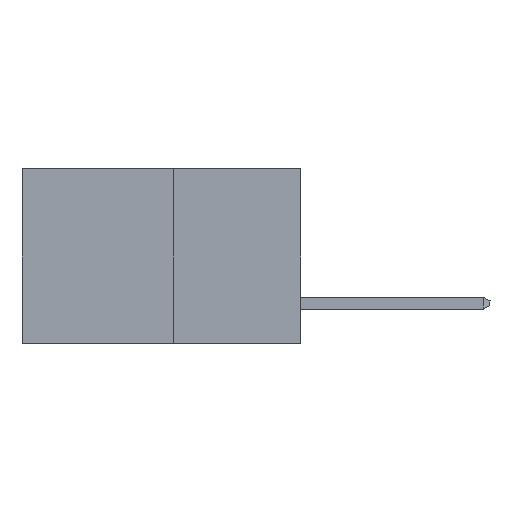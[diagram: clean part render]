
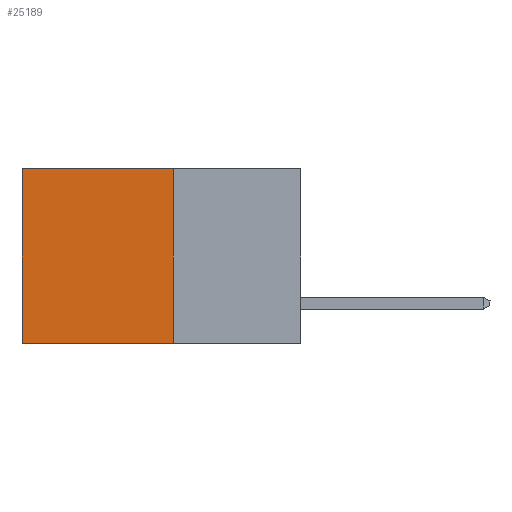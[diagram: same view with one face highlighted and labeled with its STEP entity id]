
A CAD part, left-side view. The second image highlights one B-rep face of the part: STEP entity #25189.
In plain terms, the highlighted planar face has unit normal (-1, 0, 0).
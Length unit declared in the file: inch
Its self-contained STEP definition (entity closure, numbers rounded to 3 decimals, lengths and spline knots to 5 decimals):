
#1989 = CARTESIAN_POINT ( 'NONE',  ( 0.277, 0.27, 0. ) ) ;
#2246 = VERTEX_POINT ( 'NONE', #28020 ) ;
#4218 = LINE ( 'NONE', #16928, #22026 ) ;
#4306 = LINE ( 'NONE', #18485, #16196 ) ;
#4368 = CARTESIAN_POINT ( 'NONE',  ( 0.277, 0.27, -0.37 ) ) ;
#5624 = ORIENTED_EDGE ( 'NONE', *, *, #8021, .F. ) ;
#7954 = DIRECTION ( 'NONE',  ( 0., 1., 0. ) ) ;
#8021 = EDGE_CURVE ( 'NONE', #15554, #9313, #17355, .T. ) ;
#8435 = PLANE ( 'NONE',  #23265 ) ;
#8620 = VERTEX_POINT ( 'NONE', #1989 ) ;
#9313 = VERTEX_POINT ( 'NONE', #13211 ) ;
#9419 = VECTOR ( 'NONE', #7954, 39.37008 ) ;
#10452 = CARTESIAN_POINT ( 'NONE',  ( 0.277, 0.27, -0.37 ) ) ;
#10626 = EDGE_LOOP ( 'NONE', ( #17149, #5624, #13138, #19740 ) ) ;
#10680 = CARTESIAN_POINT ( 'NONE',  ( 0.277, 0.27, -0.37 ) ) ;
#11411 = VECTOR ( 'NONE', #28932, 39.37008 ) ;
#11792 = DIRECTION ( 'NONE',  ( 0., 0., -1. ) ) ;
#12444 = DIRECTION ( 'NONE',  ( 0., 0., -1. ) ) ;
#12917 = DIRECTION ( 'NONE',  ( 1., 0., 0. ) ) ;
#13138 = ORIENTED_EDGE ( 'NONE', *, *, #14913, .F. ) ;
#13211 = CARTESIAN_POINT ( 'NONE',  ( 0.277, 0.59, -0.37 ) ) ;
#14913 = EDGE_CURVE ( 'NONE', #8620, #15554, #4218, .T. ) ;
#15338 = FACE_OUTER_BOUND ( 'NONE', #10626, .T. ) ;
#15554 = VERTEX_POINT ( 'NONE', #10452 ) ;
#16196 = VECTOR ( 'NONE', #11792, 39.37008 ) ;
#16928 = CARTESIAN_POINT ( 'NONE',  ( 0.277, 0.27, -0.37 ) ) ;
#17149 = ORIENTED_EDGE ( 'NONE', *, *, #27931, .T. ) ;
#17355 = LINE ( 'NONE', #4368, #11411 ) ;
#18485 = CARTESIAN_POINT ( 'NONE',  ( 0.277, 0.59, -0.37 ) ) ;
#19740 = ORIENTED_EDGE ( 'NONE', *, *, #21064, .T. ) ;
#20564 = LINE ( 'NONE', #25742, #9419 ) ;
#21064 = EDGE_CURVE ( 'NONE', #8620, #2246, #20564, .T. ) ;
#22026 = VECTOR ( 'NONE', #12444, 39.37008 ) ;
#23265 = AXIS2_PLACEMENT_3D ( 'NONE', #10680, #12917, #28477 ) ;
#25189 = ADVANCED_FACE ( 'NONE', ( #15338 ), #8435, .F. ) ;
#25742 = CARTESIAN_POINT ( 'NONE',  ( 0.277, 0.27, 0. ) ) ;
#27931 = EDGE_CURVE ( 'NONE', #2246, #9313, #4306, .T. ) ;
#28020 = CARTESIAN_POINT ( 'NONE',  ( 0.277, 0.59, 0. ) ) ;
#28477 = DIRECTION ( 'NONE',  ( 0., 0., -1. ) ) ;
#28932 = DIRECTION ( 'NONE',  ( 0., 1., 0. ) ) ;
